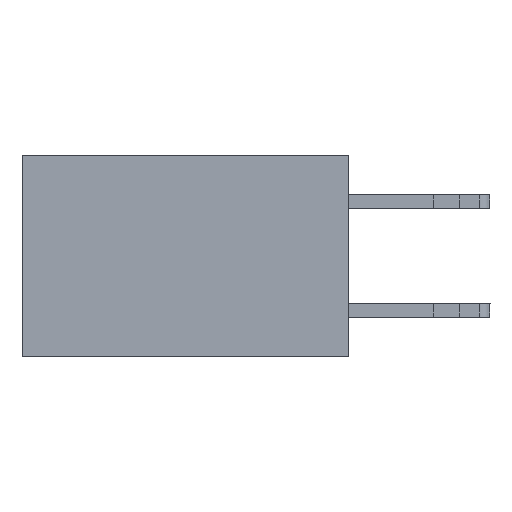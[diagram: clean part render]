
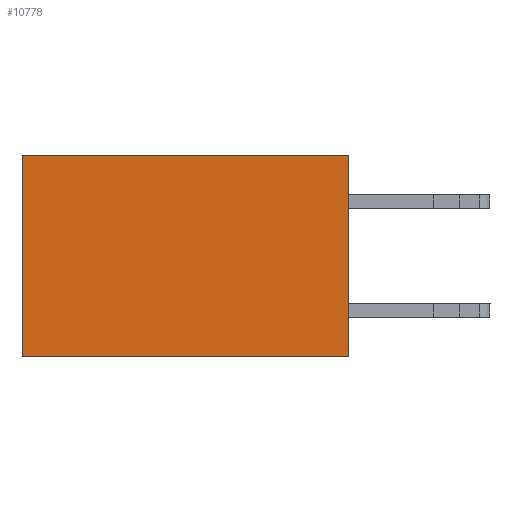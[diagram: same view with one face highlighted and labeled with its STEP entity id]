
A CAD part, left-side view. The second image highlights one B-rep face of the part: STEP entity #10778.
In plain terms, the highlighted planar face has unit normal (-1, 0, 0).
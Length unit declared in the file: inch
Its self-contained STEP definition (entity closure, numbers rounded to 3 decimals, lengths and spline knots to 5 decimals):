
#488 = CARTESIAN_POINT ( 'NONE',  ( 0.2615, 0.6, -0.37 ) ) ;
#1688 = PLANE ( 'NONE',  #13596 ) ;
#2439 = ORIENTED_EDGE ( 'NONE', *, *, #15949, .T. ) ;
#2634 = CARTESIAN_POINT ( 'NONE',  ( 0.2615, 0., 0. ) ) ;
#2994 = DIRECTION ( 'NONE',  ( 0., 0., -1. ) ) ;
#3907 = VERTEX_POINT ( 'NONE', #7266 ) ;
#4514 = CARTESIAN_POINT ( 'NONE',  ( 0.2615, 0., -0.37 ) ) ;
#4824 = FACE_OUTER_BOUND ( 'NONE', #8602, .T. ) ;
#5365 = VERTEX_POINT ( 'NONE', #15025 ) ;
#5469 = ORIENTED_EDGE ( 'NONE', *, *, #10887, .F. ) ;
#5820 = DIRECTION ( 'NONE',  ( 0., 1., 0. ) ) ;
#6100 = VECTOR ( 'NONE', #14342, 39.37008 ) ;
#7022 = DIRECTION ( 'NONE',  ( 0., 0., -1. ) ) ;
#7266 = CARTESIAN_POINT ( 'NONE',  ( 0.2615, 0., 0. ) ) ;
#8203 = CARTESIAN_POINT ( 'NONE',  ( 0.2615, 0., -0.37 ) ) ;
#8214 = VECTOR ( 'NONE', #10218, 39.37008 ) ;
#8602 = EDGE_LOOP ( 'NONE', ( #15432, #5469, #15861, #2439 ) ) ;
#8702 = EDGE_CURVE ( 'NONE', #3907, #11708, #12466, .T. ) ;
#9575 = CARTESIAN_POINT ( 'NONE',  ( 0.2615, 0.6, 0. ) ) ;
#9778 = LINE ( 'NONE', #4514, #12785 ) ;
#10205 = CARTESIAN_POINT ( 'NONE',  ( 0.2615, 0., -0.37 ) ) ;
#10218 = DIRECTION ( 'NONE',  ( 0., 0., -1. ) ) ;
#10492 = LINE ( 'NONE', #488, #13499 ) ;
#10778 = ADVANCED_FACE ( 'NONE', ( #4824 ), #1688, .F. ) ;
#10829 = DIRECTION ( 'NONE',  ( 1., 0., 0. ) ) ;
#10887 = EDGE_CURVE ( 'NONE', #11708, #5365, #9778, .T. ) ;
#11708 = VERTEX_POINT ( 'NONE', #16503 ) ;
#12466 = LINE ( 'NONE', #10205, #8214 ) ;
#12785 = VECTOR ( 'NONE', #5820, 39.37008 ) ;
#13499 = VECTOR ( 'NONE', #7022, 39.37008 ) ;
#13596 = AXIS2_PLACEMENT_3D ( 'NONE', #8203, #10829, #2994 ) ;
#14140 = EDGE_CURVE ( 'NONE', #16764, #5365, #10492, .T. ) ;
#14342 = DIRECTION ( 'NONE',  ( 0., 1., 0. ) ) ;
#15025 = CARTESIAN_POINT ( 'NONE',  ( 0.2615, 0.6, -0.37 ) ) ;
#15432 = ORIENTED_EDGE ( 'NONE', *, *, #14140, .T. ) ;
#15861 = ORIENTED_EDGE ( 'NONE', *, *, #8702, .F. ) ;
#15949 = EDGE_CURVE ( 'NONE', #3907, #16764, #16494, .T. ) ;
#16494 = LINE ( 'NONE', #2634, #6100 ) ;
#16503 = CARTESIAN_POINT ( 'NONE',  ( 0.2615, 0., -0.37 ) ) ;
#16764 = VERTEX_POINT ( 'NONE', #9575 ) ;
